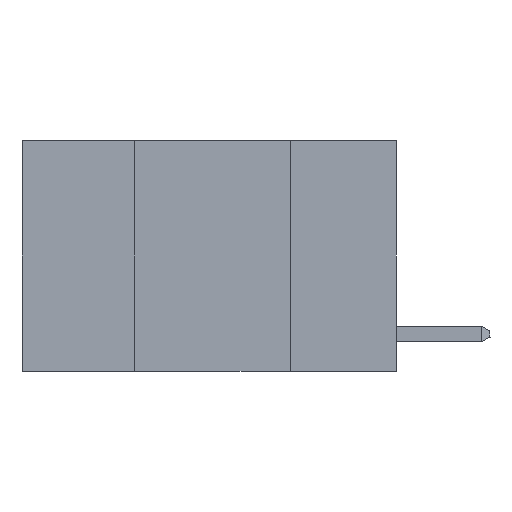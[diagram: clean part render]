
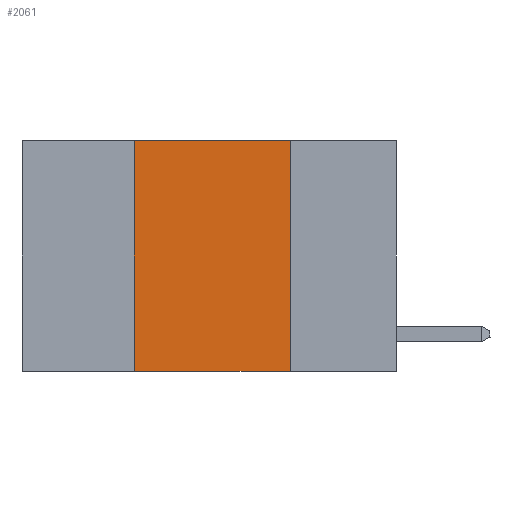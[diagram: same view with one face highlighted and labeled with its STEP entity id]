
A CAD part, left-side view. The second image highlights one B-rep face of the part: STEP entity #2061.
In plain terms, the highlighted planar face has unit normal (-1, 0, 0).
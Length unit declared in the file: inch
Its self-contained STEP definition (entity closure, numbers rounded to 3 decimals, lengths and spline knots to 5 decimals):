
#405 = VECTOR ( 'NONE', #14487, 39.37008 ) ;
#1000 = VECTOR ( 'NONE', #6898, 39.37008 ) ;
#2061 = ADVANCED_FACE ( 'NONE', ( #8931 ), #26647, .F. ) ;
#2870 = DIRECTION ( 'NONE',  ( 0., 0., 1. ) ) ;
#3007 = LINE ( 'NONE', #28316, #25666 ) ;
#3261 = LINE ( 'NONE', #16053, #8431 ) ;
#4187 = EDGE_CURVE ( 'NONE', #20000, #7519, #18581, .T. ) ;
#5158 = ORIENTED_EDGE ( 'NONE', *, *, #6288, .T. ) ;
#6055 = CARTESIAN_POINT ( 'NONE',  ( 0., 0.42, 0. ) ) ;
#6165 = LINE ( 'NONE', #20005, #1000 ) ;
#6288 = EDGE_CURVE ( 'NONE', #11263, #10604, #3007, .T. ) ;
#6898 = DIRECTION ( 'NONE',  ( 0., 0., -1. ) ) ;
#7519 = VERTEX_POINT ( 'NONE', #14229 ) ;
#8431 = VECTOR ( 'NONE', #2870, 39.37008 ) ;
#8931 = FACE_OUTER_BOUND ( 'NONE', #17409, .T. ) ;
#9244 = DIRECTION ( 'NONE',  ( 1., 0., 0. ) ) ;
#10604 = VERTEX_POINT ( 'NONE', #17971 ) ;
#11263 = VERTEX_POINT ( 'NONE', #24663 ) ;
#13369 = ORIENTED_EDGE ( 'NONE', *, *, #18034, .F. ) ;
#14229 = CARTESIAN_POINT ( 'NONE',  ( 0., 0.17, 0. ) ) ;
#14487 = DIRECTION ( 'NONE',  ( 0., -1., 0. ) ) ;
#15135 = EDGE_CURVE ( 'NONE', #11263, #20000, #3261, .T. ) ;
#15759 = ORIENTED_EDGE ( 'NONE', *, *, #4187, .F. ) ;
#15777 = CARTESIAN_POINT ( 'NONE',  ( 0., 0.6, 0. ) ) ;
#16053 = CARTESIAN_POINT ( 'NONE',  ( 0., 0.42, 0. ) ) ;
#16070 = AXIS2_PLACEMENT_3D ( 'NONE', #15777, #9244, #24588 ) ;
#17409 = EDGE_LOOP ( 'NONE', ( #13369, #15759, #19929, #5158 ) ) ;
#17431 = DIRECTION ( 'NONE',  ( 0., -1., 0. ) ) ;
#17971 = CARTESIAN_POINT ( 'NONE',  ( 0., 0.17, -0.37 ) ) ;
#18034 = EDGE_CURVE ( 'NONE', #7519, #10604, #6165, .T. ) ;
#18581 = LINE ( 'NONE', #25406, #405 ) ;
#19929 = ORIENTED_EDGE ( 'NONE', *, *, #15135, .F. ) ;
#20000 = VERTEX_POINT ( 'NONE', #6055 ) ;
#20005 = CARTESIAN_POINT ( 'NONE',  ( 0., 0.17, 0. ) ) ;
#24588 = DIRECTION ( 'NONE',  ( 0., 0., -1. ) ) ;
#24663 = CARTESIAN_POINT ( 'NONE',  ( 0., 0.42, -0.37 ) ) ;
#25406 = CARTESIAN_POINT ( 'NONE',  ( 0., 0.6, 0. ) ) ;
#25666 = VECTOR ( 'NONE', #17431, 39.37008 ) ;
#26647 = PLANE ( 'NONE',  #16070 ) ;
#28316 = CARTESIAN_POINT ( 'NONE',  ( 0., 0.6, -0.37 ) ) ;
